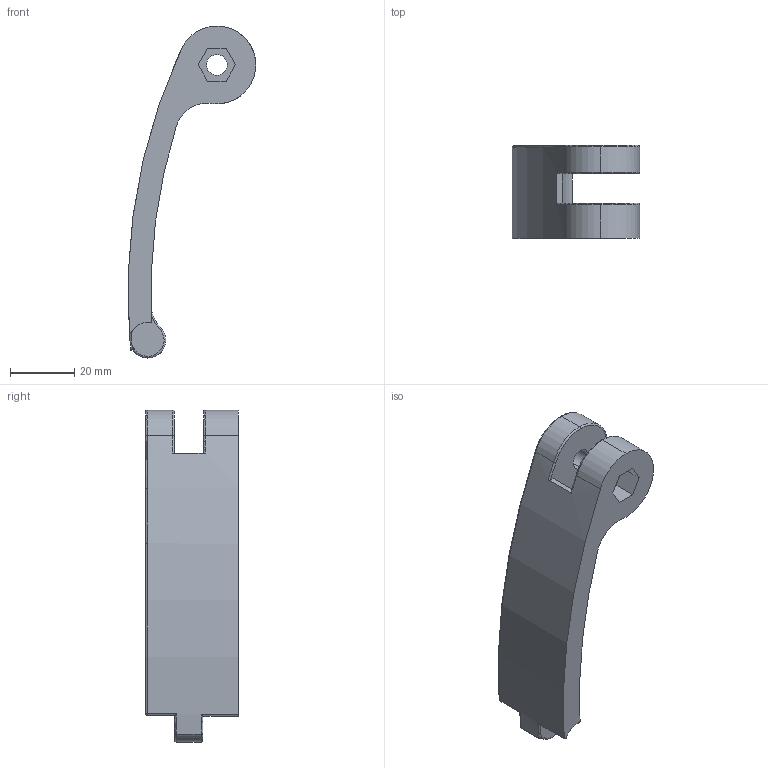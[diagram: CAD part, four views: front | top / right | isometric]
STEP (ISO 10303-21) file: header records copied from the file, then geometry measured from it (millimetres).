
FILE_DESCRIPTION (( 'STEP AP214' ), '1' );
FILE_NAME ('TailhookB.STEP', '2022-08-05T18:43:22', ( '' ), ( '' ), 'SwSTEP 2.0', 'SolidWorks 2021', '' );
FILE_SCHEMA (( 'AUTOMOTIVE_DESIGN' ));
Length unit declared in the file: millimetre
Products named in the file (1): TailhookB
Bounding box: 39.84 x 29 x 103.69 mm (x, y, z)
Volume: 25688.3 mm3; surface area: 9937.5 mm2
Topology: 1 solids, 1 shells, 87 faces, 219 edges, 133 vertices
Faces by surface type: cylinder 37, torus 30, plane 17, bspline 2, sphere 1
Entity records: 3043 total; most frequent: CARTESIAN_POINT 649, DIRECTION 492, ORIENTED_EDGE 432, EDGE_CURVE 216, AXIS2_PLACEMENT_3D 214, VERTEX_POINT 133, CIRCLE 128, EDGE_LOOP 93
